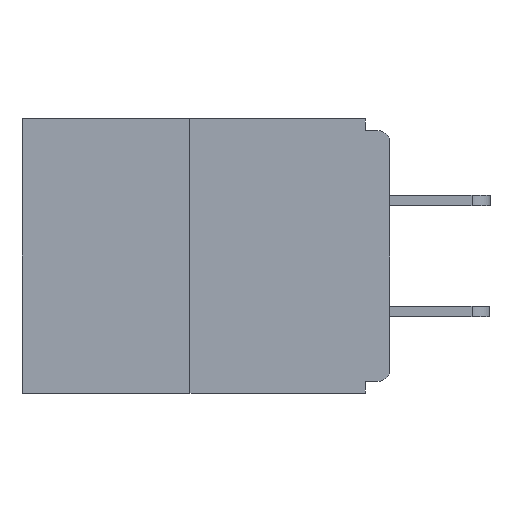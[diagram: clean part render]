
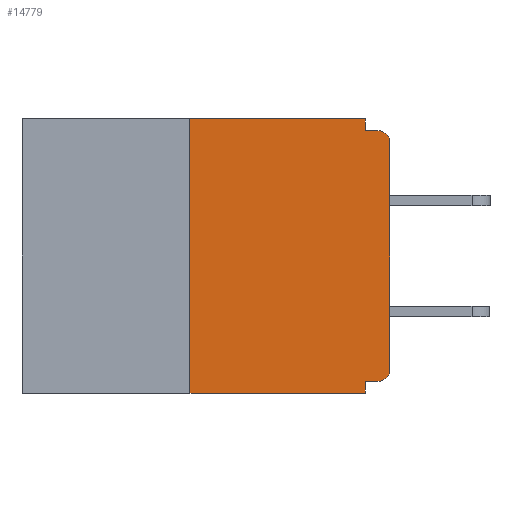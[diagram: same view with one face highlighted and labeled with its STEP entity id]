
A CAD part, left-side view. The second image highlights one B-rep face of the part: STEP entity #14779.
In plain terms, the highlighted planar face has unit normal (-1, 0, 0).
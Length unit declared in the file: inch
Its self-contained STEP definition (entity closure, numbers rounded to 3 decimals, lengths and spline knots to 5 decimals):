
#237 = DIRECTION ( 'NONE',  ( 0., -1., 0. ) ) ;
#481 = DIRECTION ( 'NONE',  ( 0., 0., -1. ) ) ;
#617 = CARTESIAN_POINT ( 'NONE',  ( 0., 0.031, 0. ) ) ;
#663 = CARTESIAN_POINT ( 'NONE',  ( 0., 0.015, -0.03 ) ) ;
#745 = EDGE_CURVE ( 'NONE', #1506, #9601, #3514, .T. ) ;
#1011 = VERTEX_POINT ( 'NONE', #16753 ) ;
#1051 = VECTOR ( 'NONE', #9066, 39.37008 ) ;
#1326 = CARTESIAN_POINT ( 'NONE',  ( 0., 0.031, 0. ) ) ;
#1506 = VERTEX_POINT ( 'NONE', #2124 ) ;
#1819 = CARTESIAN_POINT ( 'NONE',  ( 0., 0., 0. ) ) ;
#1860 = CARTESIAN_POINT ( 'NONE',  ( 0., 0.015, -0.015 ) ) ;
#1930 = CARTESIAN_POINT ( 'NONE',  ( 0., 0.015, -0.328 ) ) ;
#2124 = CARTESIAN_POINT ( 'NONE',  ( 0., 0., -0.03 ) ) ;
#2319 = ORIENTED_EDGE ( 'NONE', *, *, #4870, .F. ) ;
#2640 = CARTESIAN_POINT ( 'NONE',  ( 0., 0., -0.015 ) ) ;
#3514 = CIRCLE ( 'NONE', #7393, 0.015 ) ;
#3553 = CARTESIAN_POINT ( 'NONE',  ( 0., 0.015, -0.313 ) ) ;
#3618 = EDGE_LOOP ( 'NONE', ( #11901, #4428, #17286, #7889, #12652, #5659, #14408, #6201, #2319, #12577 ) ) ;
#3639 = CARTESIAN_POINT ( 'NONE',  ( 0., 0.031, -0.343 ) ) ;
#3803 = EDGE_CURVE ( 'NONE', #9622, #11404, #11165, .T. ) ;
#3901 = VERTEX_POINT ( 'NONE', #14936 ) ;
#4428 = ORIENTED_EDGE ( 'NONE', *, *, #10176, .F. ) ;
#4537 = LINE ( 'NONE', #7578, #6473 ) ;
#4870 = EDGE_CURVE ( 'NONE', #6659, #9601, #10906, .T. ) ;
#5223 = LINE ( 'NONE', #16821, #12564 ) ;
#5659 = ORIENTED_EDGE ( 'NONE', *, *, #3803, .T. ) ;
#5748 = VECTOR ( 'NONE', #7343, 39.37008 ) ;
#6038 = CARTESIAN_POINT ( 'NONE',  ( 0., 0., -0.328 ) ) ;
#6201 = ORIENTED_EDGE ( 'NONE', *, *, #745, .T. ) ;
#6260 = DIRECTION ( 'NONE',  ( -1., 0., 0. ) ) ;
#6437 = CARTESIAN_POINT ( 'NONE',  ( 0., 0.031, -0.343 ) ) ;
#6473 = VECTOR ( 'NONE', #9017, 39.37008 ) ;
#6659 = VERTEX_POINT ( 'NONE', #12065 ) ;
#7343 = DIRECTION ( 'NONE',  ( 0., 0., 1. ) ) ;
#7393 = AXIS2_PLACEMENT_3D ( 'NONE', #663, #11558, #481 ) ;
#7578 = CARTESIAN_POINT ( 'NONE',  ( 0., 0.46, 0. ) ) ;
#7797 = DIRECTION ( 'NONE',  ( 1., 0., 0. ) ) ;
#7889 = ORIENTED_EDGE ( 'NONE', *, *, #9653, .F. ) ;
#7908 = CARTESIAN_POINT ( 'NONE',  ( 0., 0.46, 0. ) ) ;
#8175 = CARTESIAN_POINT ( 'NONE',  ( 0., 0.25, -0.343 ) ) ;
#8360 = LINE ( 'NONE', #3639, #1051 ) ;
#8867 = CARTESIAN_POINT ( 'NONE',  ( 0., 0., -0.313 ) ) ;
#9017 = DIRECTION ( 'NONE',  ( 0., -1., 0. ) ) ;
#9066 = DIRECTION ( 'NONE',  ( 0., 0., -1. ) ) ;
#9280 = DIRECTION ( 'NONE',  ( 0., 0., -1. ) ) ;
#9329 = VERTEX_POINT ( 'NONE', #1326 ) ;
#9429 = LINE ( 'NONE', #1819, #5748 ) ;
#9601 = VERTEX_POINT ( 'NONE', #1860 ) ;
#9622 = VERTEX_POINT ( 'NONE', #1930 ) ;
#9653 = EDGE_CURVE ( 'NONE', #3901, #11652, #8360, .T. ) ;
#9835 = AXIS2_PLACEMENT_3D ( 'NONE', #7908, #7797, #9280 ) ;
#9896 = FACE_OUTER_BOUND ( 'NONE', #3618, .T. ) ;
#9982 = EDGE_CURVE ( 'NONE', #11404, #1506, #9429, .T. ) ;
#10176 = EDGE_CURVE ( 'NONE', #14487, #1011, #17247, .T. ) ;
#10264 = DIRECTION ( 'NONE',  ( 0., 1., 0. ) ) ;
#10906 = LINE ( 'NONE', #2640, #15474 ) ;
#10910 = VECTOR ( 'NONE', #17241, 39.37008 ) ;
#11150 = VECTOR ( 'NONE', #13575, 39.37008 ) ;
#11165 = CIRCLE ( 'NONE', #12773, 0.015 ) ;
#11404 = VERTEX_POINT ( 'NONE', #8867 ) ;
#11451 = EDGE_CURVE ( 'NONE', #9329, #6659, #16139, .T. ) ;
#11558 = DIRECTION ( 'NONE',  ( -1., 0., 0. ) ) ;
#11652 = VERTEX_POINT ( 'NONE', #6437 ) ;
#11901 = ORIENTED_EDGE ( 'NONE', *, *, #14187, .F. ) ;
#12065 = CARTESIAN_POINT ( 'NONE',  ( 0., 0.031, -0.015 ) ) ;
#12173 = CARTESIAN_POINT ( 'NONE',  ( 0., 0.25, 0. ) ) ;
#12371 = LINE ( 'NONE', #6038, #15634 ) ;
#12448 = EDGE_CURVE ( 'NONE', #9622, #3901, #12371, .T. ) ;
#12564 = VECTOR ( 'NONE', #14282, 39.37008 ) ;
#12577 = ORIENTED_EDGE ( 'NONE', *, *, #11451, .F. ) ;
#12652 = ORIENTED_EDGE ( 'NONE', *, *, #12448, .F. ) ;
#12661 = EDGE_CURVE ( 'NONE', #14487, #11652, #5223, .T. ) ;
#12773 = AXIS2_PLACEMENT_3D ( 'NONE', #3553, #6260, #15903 ) ;
#13575 = DIRECTION ( 'NONE',  ( 0., 0., 1. ) ) ;
#14187 = EDGE_CURVE ( 'NONE', #1011, #9329, #4537, .T. ) ;
#14282 = DIRECTION ( 'NONE',  ( 0., -1., 0. ) ) ;
#14408 = ORIENTED_EDGE ( 'NONE', *, *, #9982, .T. ) ;
#14487 = VERTEX_POINT ( 'NONE', #8175 ) ;
#14779 = ADVANCED_FACE ( 'NONE', ( #9896 ), #16153, .F. ) ;
#14936 = CARTESIAN_POINT ( 'NONE',  ( 0., 0.031, -0.328 ) ) ;
#15474 = VECTOR ( 'NONE', #237, 39.37008 ) ;
#15634 = VECTOR ( 'NONE', #10264, 39.37008 ) ;
#15903 = DIRECTION ( 'NONE',  ( 0., 0., -1. ) ) ;
#16139 = LINE ( 'NONE', #617, #10910 ) ;
#16153 = PLANE ( 'NONE',  #9835 ) ;
#16753 = CARTESIAN_POINT ( 'NONE',  ( 0., 0.25, 0. ) ) ;
#16821 = CARTESIAN_POINT ( 'NONE',  ( 0., 0.46, -0.343 ) ) ;
#17241 = DIRECTION ( 'NONE',  ( 0., 0., -1. ) ) ;
#17247 = LINE ( 'NONE', #12173, #11150 ) ;
#17286 = ORIENTED_EDGE ( 'NONE', *, *, #12661, .T. ) ;
